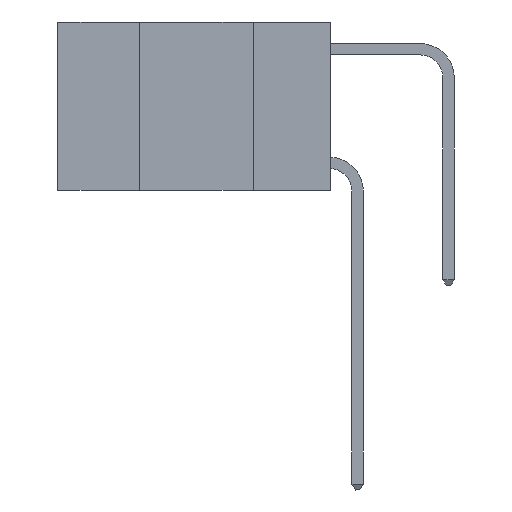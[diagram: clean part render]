
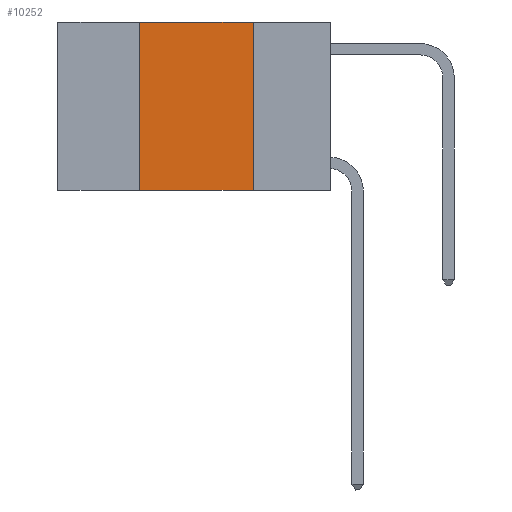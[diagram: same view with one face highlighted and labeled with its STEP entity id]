
A CAD part, left-side view. The second image highlights one B-rep face of the part: STEP entity #10252.
In plain terms, the highlighted planar face has unit normal (-1, 0, 0).
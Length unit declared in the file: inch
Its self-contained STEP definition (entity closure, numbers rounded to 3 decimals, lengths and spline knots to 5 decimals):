
#307 = CARTESIAN_POINT ( 'NONE',  ( 0., 0.42, 0. ) ) ;
#917 = ORIENTED_EDGE ( 'NONE', *, *, #6848, .T. ) ;
#976 = LINE ( 'NONE', #6548, #5619 ) ;
#990 = EDGE_CURVE ( 'NONE', #7332, #16162, #976, .T. ) ;
#1312 = CARTESIAN_POINT ( 'NONE',  ( 0., 0.6, 0. ) ) ;
#2333 = CARTESIAN_POINT ( 'NONE',  ( 0., 0.17, -0.37 ) ) ;
#2854 = DIRECTION ( 'NONE',  ( 0., -1., 0. ) ) ;
#3759 = LINE ( 'NONE', #8986, #6148 ) ;
#4473 = PLANE ( 'NONE',  #8714 ) ;
#5352 = ORIENTED_EDGE ( 'NONE', *, *, #990, .F. ) ;
#5619 = VECTOR ( 'NONE', #15693, 39.37008 ) ;
#5718 = ORIENTED_EDGE ( 'NONE', *, *, #9800, .F. ) ;
#6148 = VECTOR ( 'NONE', #19707, 39.37008 ) ;
#6205 = DIRECTION ( 'NONE',  ( 0., 0., 1. ) ) ;
#6489 = VERTEX_POINT ( 'NONE', #16131 ) ;
#6548 = CARTESIAN_POINT ( 'NONE',  ( 0., 0.17, 0. ) ) ;
#6620 = CARTESIAN_POINT ( 'NONE',  ( 0., 0.6, 0. ) ) ;
#6848 = EDGE_CURVE ( 'NONE', #7859, #16162, #3759, .T. ) ;
#7332 = VERTEX_POINT ( 'NONE', #8848 ) ;
#7859 = VERTEX_POINT ( 'NONE', #11469 ) ;
#7998 = LINE ( 'NONE', #307, #10476 ) ;
#8714 = AXIS2_PLACEMENT_3D ( 'NONE', #6620, #13736, #15766 ) ;
#8848 = CARTESIAN_POINT ( 'NONE',  ( 0., 0.17, 0. ) ) ;
#8986 = CARTESIAN_POINT ( 'NONE',  ( 0., 0.6, -0.37 ) ) ;
#9800 = EDGE_CURVE ( 'NONE', #6489, #7332, #22950, .T. ) ;
#9822 = VECTOR ( 'NONE', #2854, 39.37008 ) ;
#10252 = ADVANCED_FACE ( 'NONE', ( #15882 ), #4473, .F. ) ;
#10476 = VECTOR ( 'NONE', #6205, 39.37008 ) ;
#11469 = CARTESIAN_POINT ( 'NONE',  ( 0., 0.42, -0.37 ) ) ;
#13736 = DIRECTION ( 'NONE',  ( 1., 0., 0. ) ) ;
#15693 = DIRECTION ( 'NONE',  ( 0., 0., -1. ) ) ;
#15766 = DIRECTION ( 'NONE',  ( 0., 0., -1. ) ) ;
#15882 = FACE_OUTER_BOUND ( 'NONE', #21816, .T. ) ;
#16131 = CARTESIAN_POINT ( 'NONE',  ( 0., 0.42, 0. ) ) ;
#16162 = VERTEX_POINT ( 'NONE', #2333 ) ;
#16603 = EDGE_CURVE ( 'NONE', #7859, #6489, #7998, .T. ) ;
#19707 = DIRECTION ( 'NONE',  ( 0., -1., 0. ) ) ;
#21160 = ORIENTED_EDGE ( 'NONE', *, *, #16603, .F. ) ;
#21816 = EDGE_LOOP ( 'NONE', ( #5352, #5718, #21160, #917 ) ) ;
#22950 = LINE ( 'NONE', #1312, #9822 ) ;
